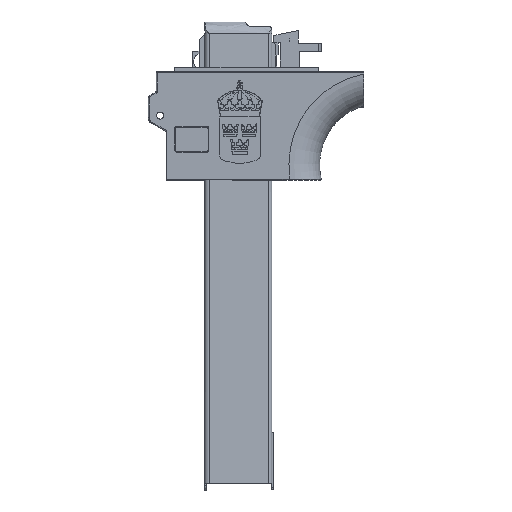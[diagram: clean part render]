
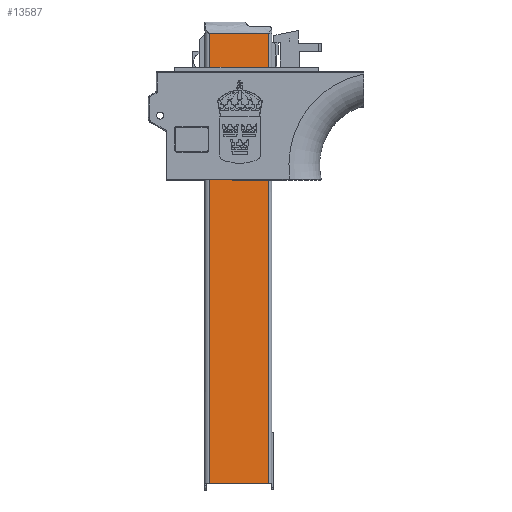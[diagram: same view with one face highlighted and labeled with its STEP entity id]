
A CAD part, top view. The second image highlights one B-rep face of the part: STEP entity #13587.
In plain terms, the highlighted planar face has unit normal (0.106, 0, 0.994).
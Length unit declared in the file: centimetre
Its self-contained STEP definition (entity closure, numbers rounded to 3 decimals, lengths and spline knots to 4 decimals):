
#1731=FACE_OUTER_BOUND($,#2518,.T.);
#2518=EDGE_LOOP($,(#11821,#11822,#11823,#11824));
#3600=LINE($,#24194,#4863);
#3685=LINE($,#25293,#4948);
#3706=LINE($,#25550,#4969);
#3709=LINE($,#25558,#4972);
#4863=VECTOR($,#16218,22.);
#4948=VECTOR($,#16331,2.9063);
#4969=VECTOR($,#16378,2.9063);
#4972=VECTOR($,#16387,22.);
#6247=VERTEX_POINT($,#24190);
#6249=VERTEX_POINT($,#24193);
#6397=VERTEX_POINT($,#25292);
#6430=VERTEX_POINT($,#25548);
#8091=EDGE_CURVE($,#6249,#6247,#3600,.T.);
#8244=EDGE_CURVE($,#6397,#6249,#3685,.T.);
#8287=EDGE_CURVE($,#6430,#6247,#3706,.T.);
#8291=EDGE_CURVE($,#6430,#6397,#3709,.T.);
#11821=ORIENTED_EDGE($,*,*,#8244,.T.);
#11822=ORIENTED_EDGE($,*,*,#8091,.T.);
#11823=ORIENTED_EDGE($,*,*,#8287,.F.);
#11824=ORIENTED_EDGE($,*,*,#8291,.T.);
#12924=PLANE($,#14254);
#13587=ADVANCED_FACE($,(#1731),#12924,.F.);
#14254=AXIS2_PLACEMENT_3D($,#25557,#16385,#16386);
#16218=DIRECTION($,(0.,-1.,0.));
#16331=DIRECTION($,(-0.994,0.,0.106));
#16378=DIRECTION($,(-0.994,0.,0.106));
#16385=DIRECTION('center_axis',(-0.106,0.,
-0.994));
#16386=DIRECTION('ref_axis',(0.994,0.,-0.106));
#16387=DIRECTION($,(0.,1.,0.));
#24190=CARTESIAN_POINT('',(-6.4003,-20.9773,1.2965));
#24193=CARTESIAN_POINT('',(-6.4003,1.0227,1.2965));
#24194=CARTESIAN_POINT($,(-6.4003,-20.9773,1.2965));
#25292=CARTESIAN_POINT('',(-3.5103,1.0227,0.989));
#25293=CARTESIAN_POINT($,(-6.6214,1.0227,1.32));
#25548=CARTESIAN_POINT('',(-3.5103,-20.9773,0.989));
#25550=CARTESIAN_POINT($,(-6.6214,-20.9773,1.32));
#25557=CARTESIAN_POINT('Origin',(-6.6214,-20.9773,1.32));
#25558=CARTESIAN_POINT($,(-3.5103,-20.9773,0.989));
